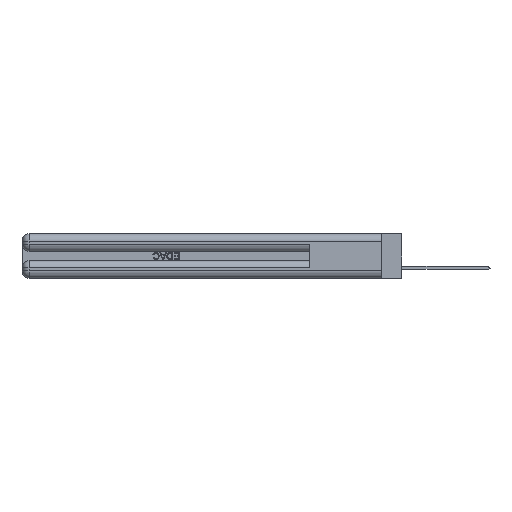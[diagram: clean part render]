
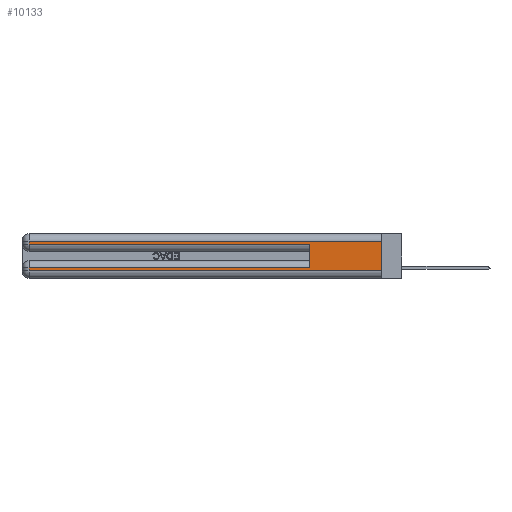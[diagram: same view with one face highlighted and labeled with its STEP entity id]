
A CAD part, left-side view. The second image highlights one B-rep face of the part: STEP entity #10133.
In plain terms, the highlighted planar face has unit normal (-1, 0, 0).
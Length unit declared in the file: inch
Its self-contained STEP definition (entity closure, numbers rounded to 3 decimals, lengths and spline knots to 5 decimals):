
#1261 = LINE ( 'NONE', #37004, #23546 ) ;
#2593 = VERTEX_POINT ( 'NONE', #24477 ) ;
#2863 = EDGE_CURVE ( 'NONE', #2593, #4446, #21289, .T. ) ;
#4099 = CARTESIAN_POINT ( 'NONE',  ( 0., 0., 0.285 ) ) ;
#4146 = CARTESIAN_POINT ( 'NONE',  ( 0., 2.94, 0.285 ) ) ;
#4446 = VERTEX_POINT ( 'NONE', #16554 ) ;
#6240 = ORIENTED_EDGE ( 'NONE', *, *, #21925, .T. ) ;
#6731 = VECTOR ( 'NONE', #42727, 39.37008 ) ;
#7345 = ORIENTED_EDGE ( 'NONE', *, *, #21085, .F. ) ;
#7533 = VERTEX_POINT ( 'NONE', #44147 ) ;
#7664 = EDGE_CURVE ( 'NONE', #8906, #7533, #24812, .T. ) ;
#8906 = VERTEX_POINT ( 'NONE', #4146 ) ;
#9455 = CARTESIAN_POINT ( 'NONE',  ( 0., 0., 0.085 ) ) ;
#10133 = ADVANCED_FACE ( 'NONE', ( #21369 ), #19421, .F. ) ;
#11436 = CARTESIAN_POINT ( 'NONE',  ( 0., 0., 0.37 ) ) ;
#11848 = DIRECTION ( 'NONE',  ( 0., 0., -1. ) ) ;
#12595 = EDGE_LOOP ( 'NONE', ( #7345, #41416, #26720, #33810, #47332, #19248, #6240, #36855 ) ) ;
#12718 = CARTESIAN_POINT ( 'NONE',  ( 0., 2.94, 0.085 ) ) ;
#14240 = VERTEX_POINT ( 'NONE', #12718 ) ;
#14395 = VECTOR ( 'NONE', #18656, 39.37008 ) ;
#14707 = CARTESIAN_POINT ( 'NONE',  ( 0., 0.6, 0.085 ) ) ;
#14943 = VECTOR ( 'NONE', #38549, 39.37008 ) ;
#15118 = VECTOR ( 'NONE', #22794, 39.37008 ) ;
#16103 = LINE ( 'NONE', #31756, #14943 ) ;
#16554 = CARTESIAN_POINT ( 'NONE',  ( 0., 0., 0.06 ) ) ;
#17113 = DIRECTION ( 'NONE',  ( 0., 1., 0. ) ) ;
#17284 = LINE ( 'NONE', #36932, #14395 ) ;
#17558 = CARTESIAN_POINT ( 'NONE',  ( 0., 0.6, 0.145 ) ) ;
#17707 = EDGE_CURVE ( 'NONE', #41670, #8906, #23898, .T. ) ;
#18656 = DIRECTION ( 'NONE',  ( 0., 1., 0. ) ) ;
#18808 = EDGE_CURVE ( 'NONE', #28015, #7533, #25009, .T. ) ;
#19248 = ORIENTED_EDGE ( 'NONE', *, *, #21359, .T. ) ;
#19421 = PLANE ( 'NONE',  #36992 ) ;
#21085 = EDGE_CURVE ( 'NONE', #31381, #4446, #1261, .T. ) ;
#21289 = LINE ( 'NONE', #41308, #25250 ) ;
#21359 = EDGE_CURVE ( 'NONE', #28015, #14240, #45966, .T. ) ;
#21369 = FACE_OUTER_BOUND ( 'NONE', #12595, .T. ) ;
#21925 = EDGE_CURVE ( 'NONE', #14240, #2593, #16103, .T. ) ;
#22699 = DIRECTION ( 'NONE',  ( 0., -1., 0. ) ) ;
#22794 = DIRECTION ( 'NONE',  ( 0., -1., 0. ) ) ;
#23080 = DIRECTION ( 'NONE',  ( 1., 0., 0. ) ) ;
#23546 = VECTOR ( 'NONE', #11848, 39.37008 ) ;
#23898 = LINE ( 'NONE', #32830, #38850 ) ;
#24477 = CARTESIAN_POINT ( 'NONE',  ( 0., 2.94, 0.06 ) ) ;
#24812 = LINE ( 'NONE', #4099, #15118 ) ;
#25009 = LINE ( 'NONE', #17558, #6731 ) ;
#25250 = VECTOR ( 'NONE', #22699, 39.37008 ) ;
#25822 = VECTOR ( 'NONE', #17113, 39.37008 ) ;
#26720 = ORIENTED_EDGE ( 'NONE', *, *, #17707, .T. ) ;
#28015 = VERTEX_POINT ( 'NONE', #14707 ) ;
#29302 = DIRECTION ( 'NONE',  ( 0., 0., -1. ) ) ;
#30298 = DIRECTION ( 'NONE',  ( 0., 0., -1. ) ) ;
#31381 = VERTEX_POINT ( 'NONE', #45284 ) ;
#31756 = CARTESIAN_POINT ( 'NONE',  ( 0., 2.94, 0.37 ) ) ;
#32830 = CARTESIAN_POINT ( 'NONE',  ( 0., 2.94, 0.37 ) ) ;
#33810 = ORIENTED_EDGE ( 'NONE', *, *, #7664, .T. ) ;
#36855 = ORIENTED_EDGE ( 'NONE', *, *, #2863, .T. ) ;
#36932 = CARTESIAN_POINT ( 'NONE',  ( 0., 0., 0.31 ) ) ;
#36992 = AXIS2_PLACEMENT_3D ( 'NONE', #11436, #23080, #30298 ) ;
#37004 = CARTESIAN_POINT ( 'NONE',  ( 0., 0., 0.37 ) ) ;
#38549 = DIRECTION ( 'NONE',  ( 0., 0., -1. ) ) ;
#38850 = VECTOR ( 'NONE', #29302, 39.37008 ) ;
#40149 = CARTESIAN_POINT ( 'NONE',  ( 0., 2.94, 0.31 ) ) ;
#41308 = CARTESIAN_POINT ( 'NONE',  ( 0., 0., 0.06 ) ) ;
#41416 = ORIENTED_EDGE ( 'NONE', *, *, #41829, .T. ) ;
#41670 = VERTEX_POINT ( 'NONE', #40149 ) ;
#41829 = EDGE_CURVE ( 'NONE', #31381, #41670, #17284, .T. ) ;
#42727 = DIRECTION ( 'NONE',  ( 0., 0., 1. ) ) ;
#44147 = CARTESIAN_POINT ( 'NONE',  ( 0., 0.6, 0.285 ) ) ;
#45284 = CARTESIAN_POINT ( 'NONE',  ( 0., 0., 0.31 ) ) ;
#45966 = LINE ( 'NONE', #9455, #25822 ) ;
#47332 = ORIENTED_EDGE ( 'NONE', *, *, #18808, .F. ) ;
